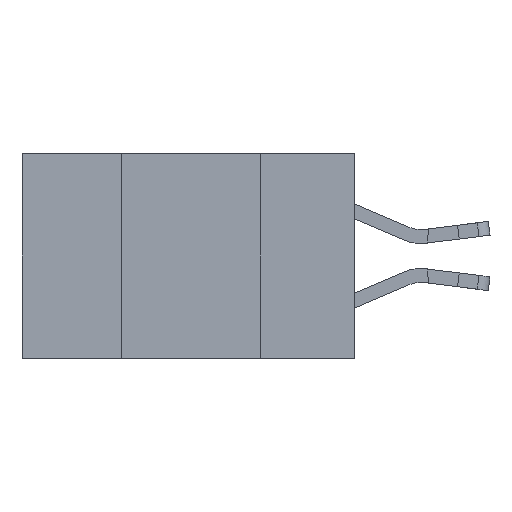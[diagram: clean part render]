
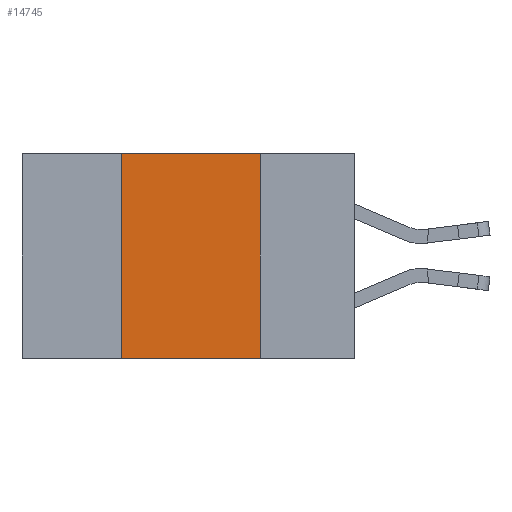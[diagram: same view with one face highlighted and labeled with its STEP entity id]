
A CAD part, left-side view. The second image highlights one B-rep face of the part: STEP entity #14745.
In plain terms, the highlighted planar face has unit normal (-1, 0, 0).
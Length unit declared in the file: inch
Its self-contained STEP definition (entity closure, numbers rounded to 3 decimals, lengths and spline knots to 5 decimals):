
#347 = AXIS2_PLACEMENT_3D ( 'NONE', #14845, #12383, #4887 ) ;
#782 = VERTEX_POINT ( 'NONE', #8917 ) ;
#1041 = VERTEX_POINT ( 'NONE', #1373 ) ;
#1373 = CARTESIAN_POINT ( 'NONE',  ( 0., 0.17, -0.37 ) ) ;
#1589 = ORIENTED_EDGE ( 'NONE', *, *, #14915, .F. ) ;
#2125 = CARTESIAN_POINT ( 'NONE',  ( 0., 0.42, -0.37 ) ) ;
#2411 = PLANE ( 'NONE',  #347 ) ;
#2731 = CARTESIAN_POINT ( 'NONE',  ( 0., 0.17, 0. ) ) ;
#3509 = EDGE_CURVE ( 'NONE', #782, #9918, #14442, .T. ) ;
#3837 = LINE ( 'NONE', #15498, #10854 ) ;
#4043 = FACE_OUTER_BOUND ( 'NONE', #9092, .T. ) ;
#4887 = DIRECTION ( 'NONE',  ( 0., 0., -1. ) ) ;
#5303 = CARTESIAN_POINT ( 'NONE',  ( 0., 0.6, 0. ) ) ;
#5316 = DIRECTION ( 'NONE',  ( 0., -1., 0. ) ) ;
#5370 = DIRECTION ( 'NONE',  ( 0., 0., 1. ) ) ;
#5682 = ORIENTED_EDGE ( 'NONE', *, *, #14071, .F. ) ;
#7432 = VECTOR ( 'NONE', #5316, 39.37008 ) ;
#7964 = VECTOR ( 'NONE', #5370, 39.37008 ) ;
#8042 = DIRECTION ( 'NONE',  ( 0., -1., 0. ) ) ;
#8335 = LINE ( 'NONE', #2731, #14552 ) ;
#8662 = ORIENTED_EDGE ( 'NONE', *, *, #3509, .F. ) ;
#8917 = CARTESIAN_POINT ( 'NONE',  ( 0., 0.42, 0. ) ) ;
#9092 = EDGE_LOOP ( 'NONE', ( #1589, #8662, #5682, #12560 ) ) ;
#9096 = CARTESIAN_POINT ( 'NONE',  ( 0., 0.17, 0. ) ) ;
#9918 = VERTEX_POINT ( 'NONE', #9096 ) ;
#10854 = VECTOR ( 'NONE', #8042, 39.37008 ) ;
#11301 = LINE ( 'NONE', #11625, #7964 ) ;
#11573 = EDGE_CURVE ( 'NONE', #14721, #1041, #3837, .T. ) ;
#11625 = CARTESIAN_POINT ( 'NONE',  ( 0., 0.42, 0. ) ) ;
#12383 = DIRECTION ( 'NONE',  ( 1., 0., 0. ) ) ;
#12560 = ORIENTED_EDGE ( 'NONE', *, *, #11573, .T. ) ;
#13904 = DIRECTION ( 'NONE',  ( 0., 0., -1. ) ) ;
#14071 = EDGE_CURVE ( 'NONE', #14721, #782, #11301, .T. ) ;
#14442 = LINE ( 'NONE', #5303, #7432 ) ;
#14552 = VECTOR ( 'NONE', #13904, 39.37008 ) ;
#14721 = VERTEX_POINT ( 'NONE', #2125 ) ;
#14745 = ADVANCED_FACE ( 'NONE', ( #4043 ), #2411, .F. ) ;
#14845 = CARTESIAN_POINT ( 'NONE',  ( 0., 0.6, 0. ) ) ;
#14915 = EDGE_CURVE ( 'NONE', #9918, #1041, #8335, .T. ) ;
#15498 = CARTESIAN_POINT ( 'NONE',  ( 0., 0.6, -0.37 ) ) ;
